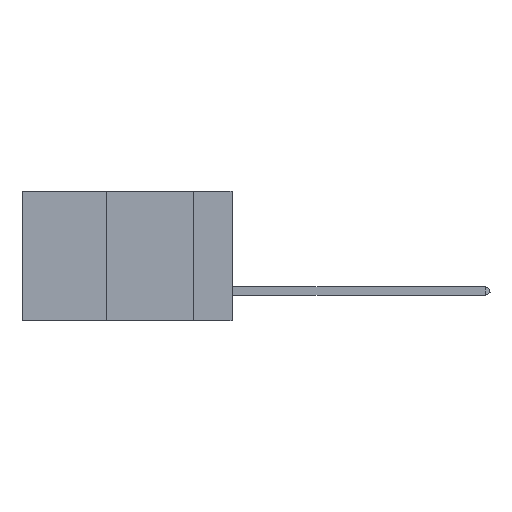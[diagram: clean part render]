
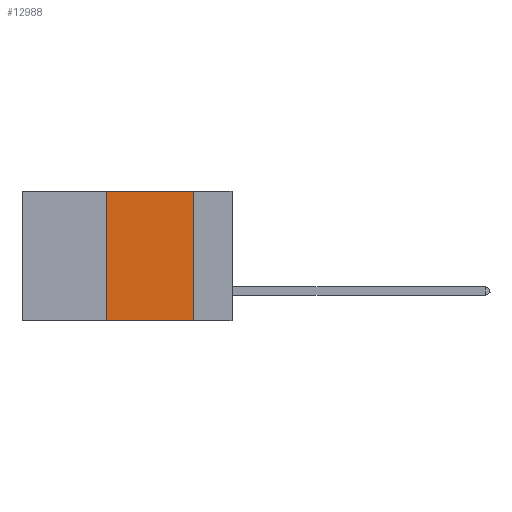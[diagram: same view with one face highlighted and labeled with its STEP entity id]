
A CAD part, left-side view. The second image highlights one B-rep face of the part: STEP entity #12988.
In plain terms, the highlighted planar face has unit normal (-1, 0, 0).
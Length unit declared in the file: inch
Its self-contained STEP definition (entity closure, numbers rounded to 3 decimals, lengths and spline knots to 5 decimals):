
#31 = CARTESIAN_POINT ( 'NONE',  ( 0., 0.11, 0. ) ) ;
#215 = ORIENTED_EDGE ( 'NONE', *, *, #9884, .F. ) ;
#688 = DIRECTION ( 'NONE',  ( 1., 0., 0. ) ) ;
#934 = EDGE_CURVE ( 'NONE', #2254, #6590, #942, .T. ) ;
#942 = LINE ( 'NONE', #1680, #3185 ) ;
#992 = VECTOR ( 'NONE', #1772, 39.37008 ) ;
#1680 = CARTESIAN_POINT ( 'NONE',  ( 0., 0.11, 0. ) ) ;
#1726 = VECTOR ( 'NONE', #2142, 39.37008 ) ;
#1772 = DIRECTION ( 'NONE',  ( 0., -1., 0. ) ) ;
#2142 = DIRECTION ( 'NONE',  ( 0., -1., 0. ) ) ;
#2254 = VERTEX_POINT ( 'NONE', #31 ) ;
#3185 = VECTOR ( 'NONE', #3742, 39.37008 ) ;
#3648 = AXIS2_PLACEMENT_3D ( 'NONE', #6718, #688, #11876 ) ;
#3742 = DIRECTION ( 'NONE',  ( 0., 0., -1. ) ) ;
#3912 = CARTESIAN_POINT ( 'NONE',  ( 0., 0.11, -0.37 ) ) ;
#4128 = ORIENTED_EDGE ( 'NONE', *, *, #12184, .T. ) ;
#4240 = VERTEX_POINT ( 'NONE', #12773 ) ;
#4406 = PLANE ( 'NONE',  #3648 ) ;
#4866 = ORIENTED_EDGE ( 'NONE', *, *, #4992, .F. ) ;
#4992 = EDGE_CURVE ( 'NONE', #4240, #10543, #10767, .T. ) ;
#5512 = FACE_OUTER_BOUND ( 'NONE', #9739, .T. ) ;
#6296 = LINE ( 'NONE', #8950, #992 ) ;
#6590 = VERTEX_POINT ( 'NONE', #3912 ) ;
#6718 = CARTESIAN_POINT ( 'NONE',  ( 0., 0.6, 0. ) ) ;
#7100 = CARTESIAN_POINT ( 'NONE',  ( 0., 0.36, 0. ) ) ;
#8375 = CARTESIAN_POINT ( 'NONE',  ( 0., 0.36, 0. ) ) ;
#8378 = VECTOR ( 'NONE', #11221, 39.37008 ) ;
#8950 = CARTESIAN_POINT ( 'NONE',  ( 0., 0.6, 0. ) ) ;
#8980 = CARTESIAN_POINT ( 'NONE',  ( 0., 0.6, -0.37 ) ) ;
#9739 = EDGE_LOOP ( 'NONE', ( #13218, #215, #4866, #4128 ) ) ;
#9884 = EDGE_CURVE ( 'NONE', #10543, #2254, #6296, .T. ) ;
#10543 = VERTEX_POINT ( 'NONE', #8375 ) ;
#10767 = LINE ( 'NONE', #7100, #8378 ) ;
#11221 = DIRECTION ( 'NONE',  ( 0., 0., 1. ) ) ;
#11876 = DIRECTION ( 'NONE',  ( 0., 0., -1. ) ) ;
#12184 = EDGE_CURVE ( 'NONE', #4240, #6590, #12593, .T. ) ;
#12593 = LINE ( 'NONE', #8980, #1726 ) ;
#12773 = CARTESIAN_POINT ( 'NONE',  ( 0., 0.36, -0.37 ) ) ;
#12988 = ADVANCED_FACE ( 'NONE', ( #5512 ), #4406, .F. ) ;
#13218 = ORIENTED_EDGE ( 'NONE', *, *, #934, .F. ) ;
